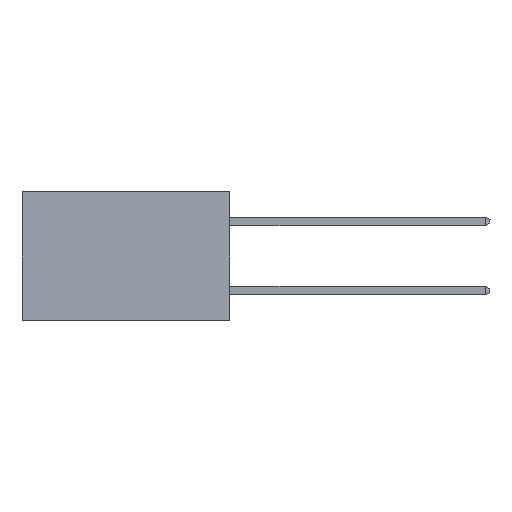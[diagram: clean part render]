
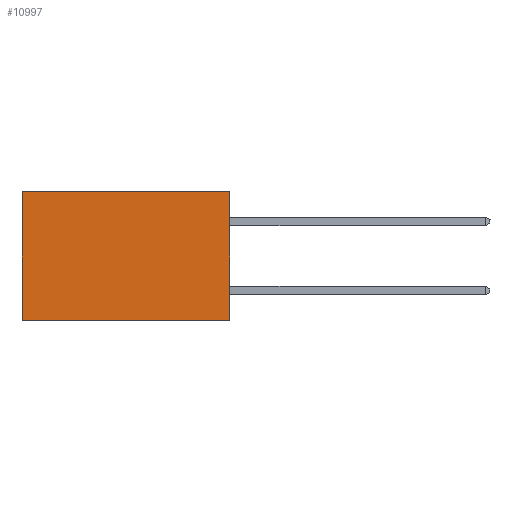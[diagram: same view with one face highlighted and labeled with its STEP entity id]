
A CAD part, left-side view. The second image highlights one B-rep face of the part: STEP entity #10997.
In plain terms, the highlighted planar face has unit normal (-1, 0, 0).
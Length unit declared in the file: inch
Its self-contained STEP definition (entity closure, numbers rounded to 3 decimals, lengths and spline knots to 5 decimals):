
#110 = CARTESIAN_POINT ( 'NONE',  ( 0.2615, 0., 0. ) ) ;
#524 = EDGE_CURVE ( 'NONE', #1181, #8277, #16065, .T. ) ;
#530 = DIRECTION ( 'NONE',  ( 0., 0., -1. ) ) ;
#1181 = VERTEX_POINT ( 'NONE', #110 ) ;
#1211 = ORIENTED_EDGE ( 'NONE', *, *, #3872, .F. ) ;
#1412 = CARTESIAN_POINT ( 'NONE',  ( 0.2615, 0., -0.37 ) ) ;
#1651 = EDGE_CURVE ( 'NONE', #10185, #15314, #6320, .T. ) ;
#2606 = DIRECTION ( 'NONE',  ( 0., 0., -1. ) ) ;
#2988 = EDGE_CURVE ( 'NONE', #1181, #10185, #9426, .T. ) ;
#3606 = DIRECTION ( 'NONE',  ( 0., 1., 0. ) ) ;
#3872 = EDGE_CURVE ( 'NONE', #8277, #15314, #7845, .T. ) ;
#4453 = CARTESIAN_POINT ( 'NONE',  ( 0.2615, 0., -0.37 ) ) ;
#5147 = CARTESIAN_POINT ( 'NONE',  ( 0.2615, 0., -0.37 ) ) ;
#5670 = VECTOR ( 'NONE', #530, 39.37008 ) ;
#5965 = CARTESIAN_POINT ( 'NONE',  ( 0.2615, 0.6, 0. ) ) ;
#6320 = LINE ( 'NONE', #11734, #5670 ) ;
#7098 = ORIENTED_EDGE ( 'NONE', *, *, #524, .F. ) ;
#7845 = LINE ( 'NONE', #5147, #9743 ) ;
#8119 = DIRECTION ( 'NONE',  ( 1., 0., 0. ) ) ;
#8277 = VERTEX_POINT ( 'NONE', #4453 ) ;
#8299 = FACE_OUTER_BOUND ( 'NONE', #11856, .T. ) ;
#9069 = CARTESIAN_POINT ( 'NONE',  ( 0.2615, 0., 0. ) ) ;
#9426 = LINE ( 'NONE', #9069, #9495 ) ;
#9495 = VECTOR ( 'NONE', #17367, 39.37008 ) ;
#9743 = VECTOR ( 'NONE', #3606, 39.37008 ) ;
#10185 = VERTEX_POINT ( 'NONE', #5965 ) ;
#10997 = ADVANCED_FACE ( 'NONE', ( #8299 ), #13789, .F. ) ;
#11734 = CARTESIAN_POINT ( 'NONE',  ( 0.2615, 0.6, -0.37 ) ) ;
#11856 = EDGE_LOOP ( 'NONE', ( #14761, #1211, #7098, #17187 ) ) ;
#11915 = DIRECTION ( 'NONE',  ( 0., 0., -1. ) ) ;
#12594 = CARTESIAN_POINT ( 'NONE',  ( 0.2615, 0.6, -0.37 ) ) ;
#13789 = PLANE ( 'NONE',  #16242 ) ;
#14155 = VECTOR ( 'NONE', #11915, 39.37008 ) ;
#14761 = ORIENTED_EDGE ( 'NONE', *, *, #1651, .T. ) ;
#15314 = VERTEX_POINT ( 'NONE', #12594 ) ;
#16065 = LINE ( 'NONE', #17529, #14155 ) ;
#16242 = AXIS2_PLACEMENT_3D ( 'NONE', #1412, #8119, #2606 ) ;
#17187 = ORIENTED_EDGE ( 'NONE', *, *, #2988, .T. ) ;
#17367 = DIRECTION ( 'NONE',  ( 0., 1., 0. ) ) ;
#17529 = CARTESIAN_POINT ( 'NONE',  ( 0.2615, 0., -0.37 ) ) ;
